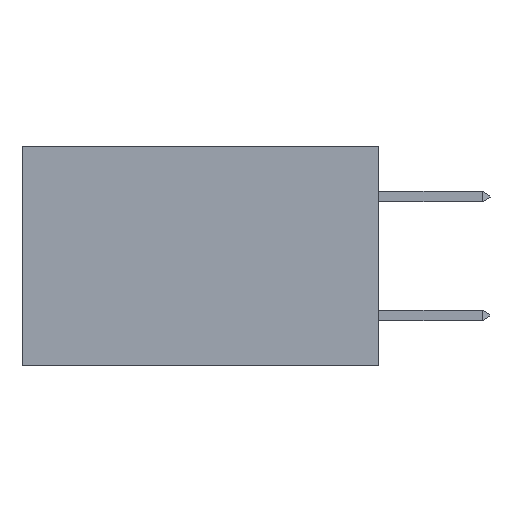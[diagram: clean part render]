
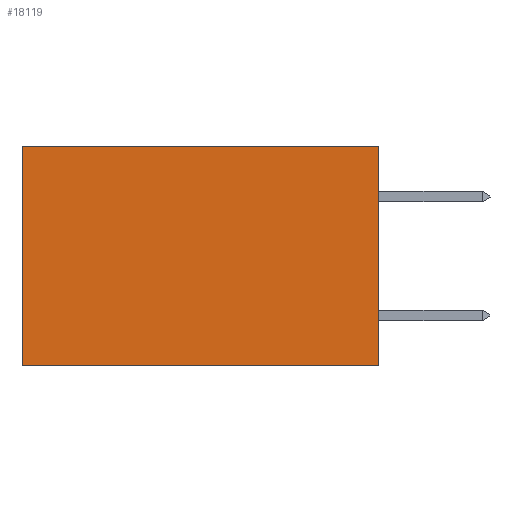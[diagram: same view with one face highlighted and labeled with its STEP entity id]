
A CAD part, left-side view. The second image highlights one B-rep face of the part: STEP entity #18119.
In plain terms, the highlighted planar face has unit normal (-1, 0, 0).
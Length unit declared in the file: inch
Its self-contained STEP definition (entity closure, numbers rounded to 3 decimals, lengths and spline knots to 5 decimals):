
#296 = LINE ( 'NONE', #11618, #22659 ) ;
#318 = EDGE_CURVE ( 'NONE', #17714, #12180, #649, .T. ) ;
#649 = LINE ( 'NONE', #5104, #23068 ) ;
#1696 = CARTESIAN_POINT ( 'NONE',  ( 0.298, 0., 0. ) ) ;
#4493 = DIRECTION ( 'NONE',  ( 1., 0., 0. ) ) ;
#4661 = ORIENTED_EDGE ( 'NONE', *, *, #318, .T. ) ;
#4723 = CARTESIAN_POINT ( 'NONE',  ( 0.298, 0., 0. ) ) ;
#5104 = CARTESIAN_POINT ( 'NONE',  ( 0.298, 0., 0. ) ) ;
#6319 = DIRECTION ( 'NONE',  ( 0., 0., -1. ) ) ;
#6988 = AXIS2_PLACEMENT_3D ( 'NONE', #4723, #4493, #9331 ) ;
#9331 = DIRECTION ( 'NONE',  ( 0., 0., -1. ) ) ;
#10040 = EDGE_CURVE ( 'NONE', #25096, #31349, #296, .T. ) ;
#11618 = CARTESIAN_POINT ( 'NONE',  ( 0.298, 0., -0.37 ) ) ;
#12180 = VERTEX_POINT ( 'NONE', #26391 ) ;
#12806 = EDGE_LOOP ( 'NONE', ( #21722, #18413, #30558, #4661 ) ) ;
#13469 = VECTOR ( 'NONE', #6319, 39.37008 ) ;
#14278 = DIRECTION ( 'NONE',  ( 0., 1., 0. ) ) ;
#15062 = FACE_OUTER_BOUND ( 'NONE', #12806, .T. ) ;
#16889 = DIRECTION ( 'NONE',  ( 0., 0., -1. ) ) ;
#17256 = PLANE ( 'NONE',  #6988 ) ;
#17714 = VERTEX_POINT ( 'NONE', #1696 ) ;
#18106 = CARTESIAN_POINT ( 'NONE',  ( 0.298, 0.6, -0.37 ) ) ;
#18119 = ADVANCED_FACE ( 'NONE', ( #15062 ), #17256, .F. ) ;
#18413 = ORIENTED_EDGE ( 'NONE', *, *, #10040, .F. ) ;
#20796 = VECTOR ( 'NONE', #16889, 39.37008 ) ;
#21722 = ORIENTED_EDGE ( 'NONE', *, *, #27369, .T. ) ;
#22659 = VECTOR ( 'NONE', #14278, 39.37008 ) ;
#23068 = VECTOR ( 'NONE', #27956, 39.37008 ) ;
#23636 = EDGE_CURVE ( 'NONE', #17714, #25096, #24209, .T. ) ;
#24209 = LINE ( 'NONE', #30909, #13469 ) ;
#25096 = VERTEX_POINT ( 'NONE', #30651 ) ;
#26391 = CARTESIAN_POINT ( 'NONE',  ( 0.298, 0.6, 0. ) ) ;
#27369 = EDGE_CURVE ( 'NONE', #12180, #31349, #29177, .T. ) ;
#27956 = DIRECTION ( 'NONE',  ( 0., 1., 0. ) ) ;
#29177 = LINE ( 'NONE', #29565, #20796 ) ;
#29565 = CARTESIAN_POINT ( 'NONE',  ( 0.298, 0.6, 0. ) ) ;
#30558 = ORIENTED_EDGE ( 'NONE', *, *, #23636, .F. ) ;
#30651 = CARTESIAN_POINT ( 'NONE',  ( 0.298, 0., -0.37 ) ) ;
#30909 = CARTESIAN_POINT ( 'NONE',  ( 0.298, 0., 0. ) ) ;
#31349 = VERTEX_POINT ( 'NONE', #18106 ) ;
